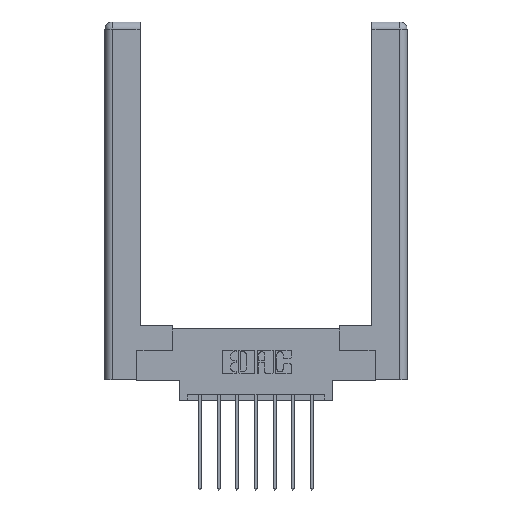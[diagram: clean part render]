
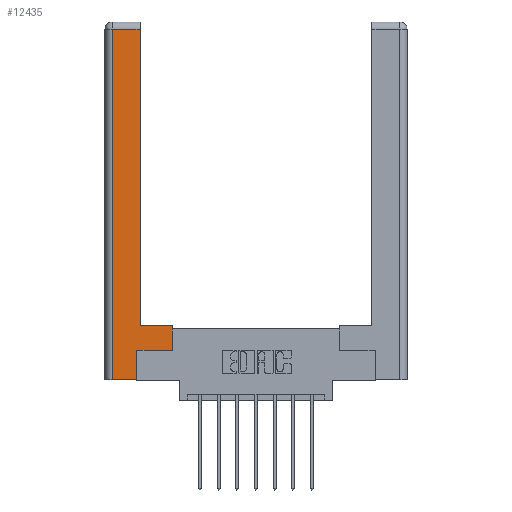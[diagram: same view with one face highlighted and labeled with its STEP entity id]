
A CAD part, top view. The second image highlights one B-rep face of the part: STEP entity #12435.
In plain terms, the highlighted planar face has unit normal (0, 0, 1).
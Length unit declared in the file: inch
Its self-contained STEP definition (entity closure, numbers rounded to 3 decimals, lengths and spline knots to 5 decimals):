
#46 = LINE ( 'NONE', #3976, #11920 ) ;
#365 = CARTESIAN_POINT ( 'NONE',  ( 0.565, 0.245, 0. ) ) ;
#605 = ORIENTED_EDGE ( 'NONE', *, *, #6309, .T. ) ;
#710 = CARTESIAN_POINT ( 'NONE',  ( 0.565, 0.245, 0. ) ) ;
#799 = VECTOR ( 'NONE', #8750, 39.37008 ) ;
#831 = CARTESIAN_POINT ( 'NONE',  ( 0.265, 0., 0. ) ) ;
#883 = ORIENTED_EDGE ( 'NONE', *, *, #8900, .T. ) ;
#1206 = VECTOR ( 'NONE', #4863, 39.37008 ) ;
#1532 = DIRECTION ( 'NONE',  ( -1., 0., 0. ) ) ;
#1662 = CARTESIAN_POINT ( 'NONE',  ( 0.265, 0.245, 0. ) ) ;
#1726 = ORIENTED_EDGE ( 'NONE', *, *, #5229, .T. ) ;
#1908 = EDGE_LOOP ( 'NONE', ( #9681, #605, #9859, #3918, #883, #6535, #1726, #3127 ) ) ;
#2782 = DIRECTION ( 'NONE',  ( 1., 0., 0. ) ) ;
#2916 = DIRECTION ( 'NONE',  ( 0., 0., -1. ) ) ;
#3127 = ORIENTED_EDGE ( 'NONE', *, *, #5885, .T. ) ;
#3227 = LINE ( 'NONE', #5305, #9861 ) ;
#3416 = CARTESIAN_POINT ( 'NONE',  ( 0.565, 0.45, 0. ) ) ;
#3579 = AXIS2_PLACEMENT_3D ( 'NONE', #4034, #2916, #10909 ) ;
#3918 = ORIENTED_EDGE ( 'NONE', *, *, #8321, .T. ) ;
#3959 = CARTESIAN_POINT ( 'NONE',  ( 0.0615, 2.94, 0. ) ) ;
#3976 = CARTESIAN_POINT ( 'NONE',  ( 0.265, 0., 0. ) ) ;
#4034 = CARTESIAN_POINT ( 'NONE',  ( 0., 0., 0. ) ) ;
#4157 = LINE ( 'NONE', #3959, #1206 ) ;
#4307 = CARTESIAN_POINT ( 'NONE',  ( 0.295, 2.94, 0. ) ) ;
#4617 = VECTOR ( 'NONE', #6060, 39.37008 ) ;
#4664 = LINE ( 'NONE', #710, #11263 ) ;
#4863 = DIRECTION ( 'NONE',  ( -1., 0., 0. ) ) ;
#5229 = EDGE_CURVE ( 'NONE', #5310, #5588, #10952, .T. ) ;
#5305 = CARTESIAN_POINT ( 'NONE',  ( 0.0615, 0., 0. ) ) ;
#5310 = VERTEX_POINT ( 'NONE', #365 ) ;
#5349 = DIRECTION ( 'NONE',  ( 0., 1., 0. ) ) ;
#5588 = VERTEX_POINT ( 'NONE', #9883 ) ;
#5885 = EDGE_CURVE ( 'NONE', #5588, #11034, #10183, .T. ) ;
#6012 = PLANE ( 'NONE',  #3579 ) ;
#6060 = DIRECTION ( 'NONE',  ( 0., 1., 0. ) ) ;
#6089 = EDGE_CURVE ( 'NONE', #8186, #7215, #3227, .T. ) ;
#6309 = EDGE_CURVE ( 'NONE', #10272, #8186, #4157, .T. ) ;
#6535 = ORIENTED_EDGE ( 'NONE', *, *, #9511, .T. ) ;
#6914 = VECTOR ( 'NONE', #1532, 39.37008 ) ;
#6972 = VERTEX_POINT ( 'NONE', #831 ) ;
#7215 = VERTEX_POINT ( 'NONE', #7634 ) ;
#7402 = VECTOR ( 'NONE', #5349, 39.37008 ) ;
#7441 = CARTESIAN_POINT ( 'NONE',  ( 0.295, 0.45, 0. ) ) ;
#7634 = CARTESIAN_POINT ( 'NONE',  ( 0.0615, 0., 0. ) ) ;
#7992 = DIRECTION ( 'NONE',  ( 0., -1., 0. ) ) ;
#8066 = CARTESIAN_POINT ( 'NONE',  ( 0.295, 0.45, 0. ) ) ;
#8186 = VERTEX_POINT ( 'NONE', #12358 ) ;
#8321 = EDGE_CURVE ( 'NONE', #7215, #6972, #46, .T. ) ;
#8702 = LINE ( 'NONE', #1662, #799 ) ;
#8750 = DIRECTION ( 'NONE',  ( 0., 1., 0. ) ) ;
#8900 = EDGE_CURVE ( 'NONE', #6972, #12507, #8702, .T. ) ;
#9019 = DIRECTION ( 'NONE',  ( 1., 0., 0. ) ) ;
#9511 = EDGE_CURVE ( 'NONE', #12507, #5310, #4664, .T. ) ;
#9681 = ORIENTED_EDGE ( 'NONE', *, *, #12426, .T. ) ;
#9859 = ORIENTED_EDGE ( 'NONE', *, *, #6089, .T. ) ;
#9861 = VECTOR ( 'NONE', #7992, 39.37008 ) ;
#9883 = CARTESIAN_POINT ( 'NONE',  ( 0.565, 0.45, 0. ) ) ;
#9955 = CARTESIAN_POINT ( 'NONE',  ( 0.295, 3., 0. ) ) ;
#10159 = CARTESIAN_POINT ( 'NONE',  ( 0.265, 0.245, 0. ) ) ;
#10183 = LINE ( 'NONE', #7441, #6914 ) ;
#10272 = VERTEX_POINT ( 'NONE', #4307 ) ;
#10909 = DIRECTION ( 'NONE',  ( -1., 0., 0. ) ) ;
#10921 = LINE ( 'NONE', #9955, #4617 ) ;
#10952 = LINE ( 'NONE', #3416, #7402 ) ;
#11034 = VERTEX_POINT ( 'NONE', #8066 ) ;
#11263 = VECTOR ( 'NONE', #2782, 39.37008 ) ;
#11544 = FACE_OUTER_BOUND ( 'NONE', #1908, .T. ) ;
#11920 = VECTOR ( 'NONE', #9019, 39.37008 ) ;
#12358 = CARTESIAN_POINT ( 'NONE',  ( 0.0615, 2.94, 0. ) ) ;
#12426 = EDGE_CURVE ( 'NONE', #11034, #10272, #10921, .T. ) ;
#12435 = ADVANCED_FACE ( 'NONE', ( #11544 ), #6012, .F. ) ;
#12507 = VERTEX_POINT ( 'NONE', #10159 ) ;
